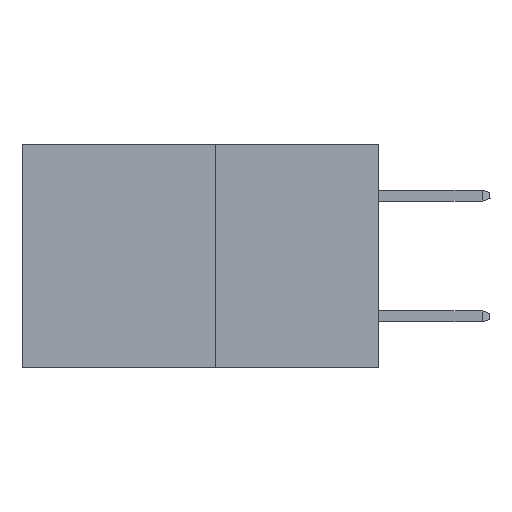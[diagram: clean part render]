
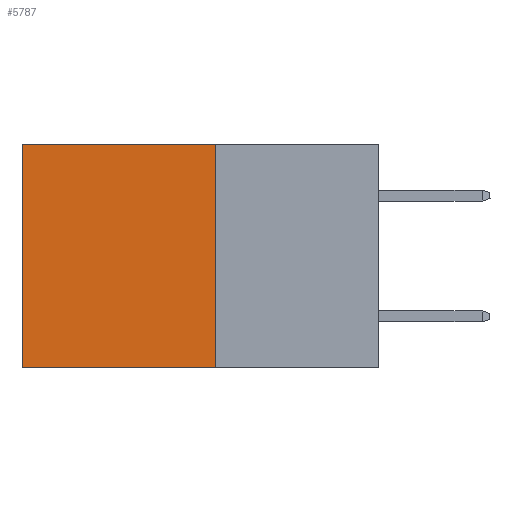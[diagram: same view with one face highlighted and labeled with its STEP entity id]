
A CAD part, left-side view. The second image highlights one B-rep face of the part: STEP entity #5787.
In plain terms, the highlighted planar face has unit normal (-1, 0, 0).
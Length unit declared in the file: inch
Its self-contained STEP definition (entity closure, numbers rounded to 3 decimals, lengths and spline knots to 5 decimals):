
#415 = VECTOR ( 'NONE', #6551, 39.37008 ) ;
#578 = DIRECTION ( 'NONE',  ( 0., 1., 0. ) ) ;
#1285 = CARTESIAN_POINT ( 'NONE',  ( 0.277, 0.27, 0. ) ) ;
#1679 = CARTESIAN_POINT ( 'NONE',  ( 0.277, 0.27, -0.37 ) ) ;
#2029 = VERTEX_POINT ( 'NONE', #1679 ) ;
#2259 = PLANE ( 'NONE',  #9248 ) ;
#3216 = VECTOR ( 'NONE', #12573, 39.37008 ) ;
#3651 = LINE ( 'NONE', #1285, #3216 ) ;
#4135 = DIRECTION ( 'NONE',  ( 0., 0., -1. ) ) ;
#4519 = LINE ( 'NONE', #9042, #7846 ) ;
#4800 = EDGE_CURVE ( 'NONE', #11929, #12669, #7880, .T. ) ;
#5039 = CARTESIAN_POINT ( 'NONE',  ( 0.277, 0.59, 0. ) ) ;
#5090 = DIRECTION ( 'NONE',  ( 0., 0., -1. ) ) ;
#5170 = ORIENTED_EDGE ( 'NONE', *, *, #9276, .F. ) ;
#5181 = LINE ( 'NONE', #13969, #15834 ) ;
#5787 = ADVANCED_FACE ( 'NONE', ( #17718 ), #2259, .F. ) ;
#5992 = EDGE_CURVE ( 'NONE', #16914, #11929, #3651, .T. ) ;
#6551 = DIRECTION ( 'NONE',  ( 0., 0., -1. ) ) ;
#6608 = EDGE_CURVE ( 'NONE', #16914, #2029, #5181, .T. ) ;
#6614 = CARTESIAN_POINT ( 'NONE',  ( 0.277, 0.59, -0.37 ) ) ;
#6946 = ORIENTED_EDGE ( 'NONE', *, *, #6608, .F. ) ;
#7846 = VECTOR ( 'NONE', #578, 39.37008 ) ;
#7880 = LINE ( 'NONE', #6614, #415 ) ;
#9042 = CARTESIAN_POINT ( 'NONE',  ( 0.277, 0.27, -0.37 ) ) ;
#9248 = AXIS2_PLACEMENT_3D ( 'NONE', #12153, #13526, #5090 ) ;
#9276 = EDGE_CURVE ( 'NONE', #2029, #12669, #4519, .T. ) ;
#10007 = CARTESIAN_POINT ( 'NONE',  ( 0.277, 0.27, 0. ) ) ;
#11929 = VERTEX_POINT ( 'NONE', #5039 ) ;
#12153 = CARTESIAN_POINT ( 'NONE',  ( 0.277, 0.27, -0.37 ) ) ;
#12573 = DIRECTION ( 'NONE',  ( 0., 1., 0. ) ) ;
#12669 = VERTEX_POINT ( 'NONE', #16511 ) ;
#13526 = DIRECTION ( 'NONE',  ( 1., 0., 0. ) ) ;
#13969 = CARTESIAN_POINT ( 'NONE',  ( 0.277, 0.27, -0.37 ) ) ;
#14355 = EDGE_LOOP ( 'NONE', ( #17466, #5170, #6946, #14597 ) ) ;
#14597 = ORIENTED_EDGE ( 'NONE', *, *, #5992, .T. ) ;
#15834 = VECTOR ( 'NONE', #4135, 39.37008 ) ;
#16511 = CARTESIAN_POINT ( 'NONE',  ( 0.277, 0.59, -0.37 ) ) ;
#16914 = VERTEX_POINT ( 'NONE', #10007 ) ;
#17466 = ORIENTED_EDGE ( 'NONE', *, *, #4800, .T. ) ;
#17718 = FACE_OUTER_BOUND ( 'NONE', #14355, .T. ) ;
